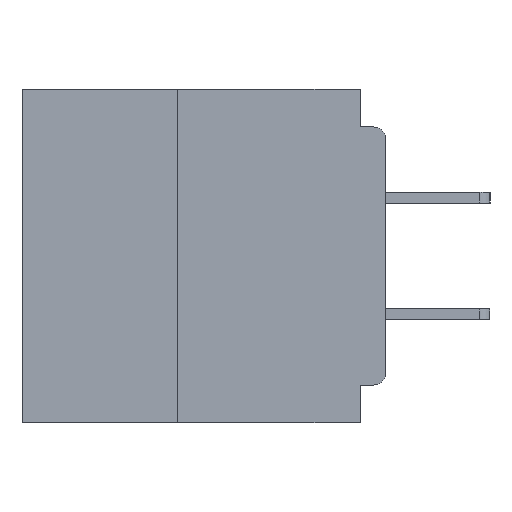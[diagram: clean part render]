
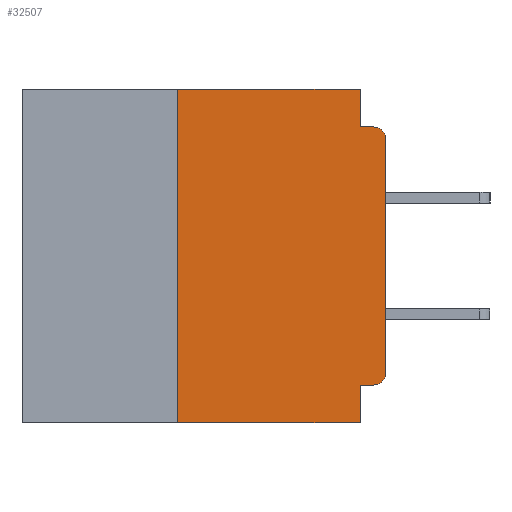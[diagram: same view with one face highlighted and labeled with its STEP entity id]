
A CAD part, left-side view. The second image highlights one B-rep face of the part: STEP entity #32507.
In plain terms, the highlighted planar face has unit normal (-1, 0, 0).
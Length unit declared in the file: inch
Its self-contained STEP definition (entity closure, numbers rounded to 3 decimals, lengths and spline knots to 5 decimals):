
#115 = LINE ( 'NONE', #16153, #7682 ) ;
#320 = CARTESIAN_POINT ( 'NONE',  ( 0., 0.031, -0.045 ) ) ;
#840 = CARTESIAN_POINT ( 'NONE',  ( 0., 0., -0.355 ) ) ;
#1747 = EDGE_CURVE ( 'NONE', #20221, #34411, #26878, .T. ) ;
#2532 = CARTESIAN_POINT ( 'NONE',  ( 0., 0., -0.045 ) ) ;
#4078 = DIRECTION ( 'NONE',  ( 0., 1., 0. ) ) ;
#4156 = CARTESIAN_POINT ( 'NONE',  ( 0., 0.031, -0.4 ) ) ;
#4471 = ORIENTED_EDGE ( 'NONE', *, *, #40213, .T. ) ;
#4501 = FACE_OUTER_BOUND ( 'NONE', #24904, .T. ) ;
#4539 = VECTOR ( 'NONE', #5764, 39.37008 ) ;
#4763 = CARTESIAN_POINT ( 'NONE',  ( 0., 0., -0.06 ) ) ;
#4887 = ORIENTED_EDGE ( 'NONE', *, *, #16443, .T. ) ;
#5116 = CARTESIAN_POINT ( 'NONE',  ( 0., 0.25, -0.4 ) ) ;
#5265 = VECTOR ( 'NONE', #17090, 39.37008 ) ;
#5764 = DIRECTION ( 'NONE',  ( 0., -1., 0. ) ) ;
#6542 = CARTESIAN_POINT ( 'NONE',  ( 0., 0.437, 0. ) ) ;
#6852 = VECTOR ( 'NONE', #4078, 39.37008 ) ;
#7543 = EDGE_CURVE ( 'NONE', #37917, #20221, #16657, .T. ) ;
#7682 = VECTOR ( 'NONE', #38526, 39.37008 ) ;
#9812 = VERTEX_POINT ( 'NONE', #5116 ) ;
#9988 = CARTESIAN_POINT ( 'NONE',  ( 0., 0.015, -0.34 ) ) ;
#10079 = EDGE_CURVE ( 'NONE', #13081, #17748, #27839, .T. ) ;
#10354 = VERTEX_POINT ( 'NONE', #30894 ) ;
#10597 = CARTESIAN_POINT ( 'NONE',  ( 0., 0.25, -0.4 ) ) ;
#12146 = VERTEX_POINT ( 'NONE', #30335 ) ;
#12217 = DIRECTION ( 'NONE',  ( 0., 0., -1. ) ) ;
#12259 = CARTESIAN_POINT ( 'NONE',  ( 0., 0.031, -0.355 ) ) ;
#12335 = EDGE_CURVE ( 'NONE', #34411, #17748, #22642, .T. ) ;
#12653 = DIRECTION ( 'NONE',  ( 1., 0., 0. ) ) ;
#12979 = DIRECTION ( 'NONE',  ( -1., 0., 0. ) ) ;
#13081 = VERTEX_POINT ( 'NONE', #4763 ) ;
#13232 = DIRECTION ( 'NONE',  ( 0., 0., -1. ) ) ;
#13621 = EDGE_CURVE ( 'NONE', #39490, #12146, #25497, .T. ) ;
#13839 = VECTOR ( 'NONE', #26480, 39.37008 ) ;
#14051 = ORIENTED_EDGE ( 'NONE', *, *, #15376, .T. ) ;
#14109 = CARTESIAN_POINT ( 'NONE',  ( 0., 0.031, 0. ) ) ;
#14119 = CARTESIAN_POINT ( 'NONE',  ( 0., 0.015, -0.045 ) ) ;
#14277 = CIRCLE ( 'NONE', #20001, 0.015 ) ;
#14734 = EDGE_CURVE ( 'NONE', #19870, #39490, #25907, .T. ) ;
#15376 = EDGE_CURVE ( 'NONE', #10354, #13081, #22368, .T. ) ;
#16153 = CARTESIAN_POINT ( 'NONE',  ( 0., 0.437, -0.4 ) ) ;
#16443 = EDGE_CURVE ( 'NONE', #19870, #10354, #14277, .T. ) ;
#16657 = LINE ( 'NONE', #6542, #23159 ) ;
#17090 = DIRECTION ( 'NONE',  ( 0., 0., 1. ) ) ;
#17748 = VERTEX_POINT ( 'NONE', #14119 ) ;
#19108 = CARTESIAN_POINT ( 'NONE',  ( 0., 0.437, 0. ) ) ;
#19870 = VERTEX_POINT ( 'NONE', #40326 ) ;
#20001 = AXIS2_PLACEMENT_3D ( 'NONE', #9988, #32434, #13232 ) ;
#20186 = DIRECTION ( 'NONE',  ( 0., 0., -1. ) ) ;
#20221 = VERTEX_POINT ( 'NONE', #36554 ) ;
#20610 = ORIENTED_EDGE ( 'NONE', *, *, #13621, .F. ) ;
#22347 = PLANE ( 'NONE',  #30741 ) ;
#22368 = LINE ( 'NONE', #23283, #13839 ) ;
#22642 = LINE ( 'NONE', #2532, #4539 ) ;
#23159 = VECTOR ( 'NONE', #28980, 39.37008 ) ;
#23266 = ORIENTED_EDGE ( 'NONE', *, *, #7543, .F. ) ;
#23283 = CARTESIAN_POINT ( 'NONE',  ( 0., 0., 0. ) ) ;
#24904 = EDGE_LOOP ( 'NONE', ( #14051, #27648, #28253, #28992, #23266, #32866, #4471, #20610, #34168, #4887 ) ) ;
#25497 = LINE ( 'NONE', #4156, #33052 ) ;
#25528 = DIRECTION ( 'NONE',  ( 0., 0., -1. ) ) ;
#25907 = LINE ( 'NONE', #840, #6852 ) ;
#26480 = DIRECTION ( 'NONE',  ( 0., 0., 1. ) ) ;
#26878 = LINE ( 'NONE', #14109, #34386 ) ;
#27648 = ORIENTED_EDGE ( 'NONE', *, *, #10079, .T. ) ;
#27839 = CIRCLE ( 'NONE', #33326, 0.015 ) ;
#28253 = ORIENTED_EDGE ( 'NONE', *, *, #12335, .F. ) ;
#28980 = DIRECTION ( 'NONE',  ( 0., -1., 0. ) ) ;
#28992 = ORIENTED_EDGE ( 'NONE', *, *, #1747, .F. ) ;
#30335 = CARTESIAN_POINT ( 'NONE',  ( 0., 0.031, -0.4 ) ) ;
#30741 = AXIS2_PLACEMENT_3D ( 'NONE', #19108, #12653, #25528 ) ;
#30894 = CARTESIAN_POINT ( 'NONE',  ( 0., 0., -0.34 ) ) ;
#32170 = CARTESIAN_POINT ( 'NONE',  ( 0., 0.015, -0.06 ) ) ;
#32434 = DIRECTION ( 'NONE',  ( -1., 0., 0. ) ) ;
#32507 = ADVANCED_FACE ( 'NONE', ( #4501 ), #22347, .F. ) ;
#32866 = ORIENTED_EDGE ( 'NONE', *, *, #39172, .F. ) ;
#33052 = VECTOR ( 'NONE', #20186, 39.37008 ) ;
#33326 = AXIS2_PLACEMENT_3D ( 'NONE', #32170, #12979, #35368 ) ;
#34141 = CARTESIAN_POINT ( 'NONE',  ( 0., 0.25, 0. ) ) ;
#34168 = ORIENTED_EDGE ( 'NONE', *, *, #14734, .F. ) ;
#34386 = VECTOR ( 'NONE', #12217, 39.37008 ) ;
#34411 = VERTEX_POINT ( 'NONE', #320 ) ;
#35368 = DIRECTION ( 'NONE',  ( 0., 0., -1. ) ) ;
#36554 = CARTESIAN_POINT ( 'NONE',  ( 0., 0.031, 0. ) ) ;
#37917 = VERTEX_POINT ( 'NONE', #34141 ) ;
#38526 = DIRECTION ( 'NONE',  ( 0., -1., 0. ) ) ;
#39172 = EDGE_CURVE ( 'NONE', #9812, #37917, #39353, .T. ) ;
#39353 = LINE ( 'NONE', #10597, #5265 ) ;
#39490 = VERTEX_POINT ( 'NONE', #12259 ) ;
#40213 = EDGE_CURVE ( 'NONE', #9812, #12146, #115, .T. ) ;
#40326 = CARTESIAN_POINT ( 'NONE',  ( 0., 0.015, -0.355 ) ) ;
